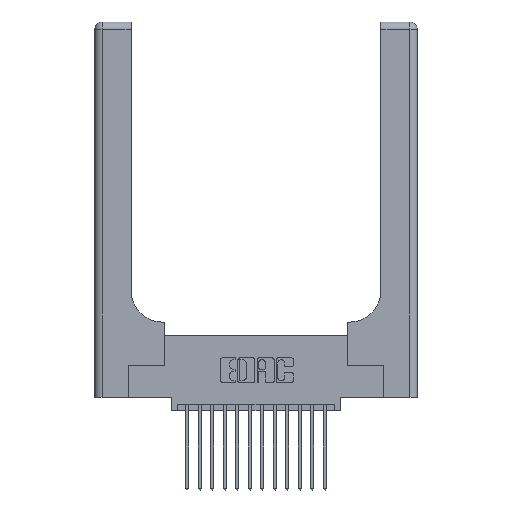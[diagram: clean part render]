
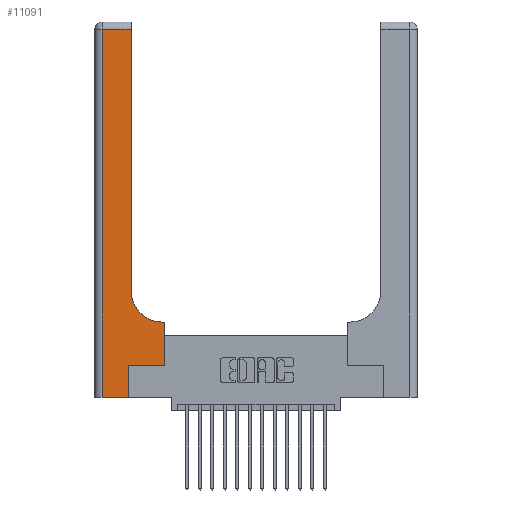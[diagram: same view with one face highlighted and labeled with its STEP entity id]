
A CAD part, top view. The second image highlights one B-rep face of the part: STEP entity #11091.
In plain terms, the highlighted planar face has unit normal (0, 0, 1).
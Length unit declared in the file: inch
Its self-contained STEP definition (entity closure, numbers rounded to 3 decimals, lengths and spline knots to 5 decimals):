
#57 = LINE ( 'NONE', #12612, #15238 ) ;
#309 = LINE ( 'NONE', #1431, #12559 ) ;
#546 = DIRECTION ( 'NONE',  ( -1., 0., 0. ) ) ;
#601 = CARTESIAN_POINT ( 'NONE',  ( 0.06, 0., 0.37 ) ) ;
#1431 = CARTESIAN_POINT ( 'NONE',  ( 0., 0., 0.37 ) ) ;
#1737 = LINE ( 'NONE', #11114, #10131 ) ;
#2006 = VERTEX_POINT ( 'NONE', #17829 ) ;
#2200 = VECTOR ( 'NONE', #17034, 39.37008 ) ;
#2235 = VECTOR ( 'NONE', #14270, 39.37008 ) ;
#2301 = VERTEX_POINT ( 'NONE', #14633 ) ;
#2372 = DIRECTION ( 'NONE',  ( -1., 0., 0. ) ) ;
#2951 = CARTESIAN_POINT ( 'NONE',  ( 0.5415, 0.85, 0.37 ) ) ;
#3018 = VECTOR ( 'NONE', #6677, 39.37008 ) ;
#3206 = ORIENTED_EDGE ( 'NONE', *, *, #6634, .T. ) ;
#3390 = CARTESIAN_POINT ( 'NONE',  ( 0.2915, 3., 0.37 ) ) ;
#3450 = AXIS2_PLACEMENT_3D ( 'NONE', #2951, #13175, #4535 ) ;
#3477 = ORIENTED_EDGE ( 'NONE', *, *, #6862, .T. ) ;
#3519 = LINE ( 'NONE', #5178, #3018 ) ;
#4175 = CARTESIAN_POINT ( 'NONE',  ( 0., 2.94, 0.37 ) ) ;
#4234 = LINE ( 'NONE', #3390, #4718 ) ;
#4363 = EDGE_CURVE ( 'NONE', #2301, #14396, #9798, .T. ) ;
#4377 = AXIS2_PLACEMENT_3D ( 'NONE', #17918, #9528, #546 ) ;
#4535 = DIRECTION ( 'NONE',  ( 1., 0., 0. ) ) ;
#4718 = VECTOR ( 'NONE', #12140, 39.37008 ) ;
#5178 = CARTESIAN_POINT ( 'NONE',  ( 0.269, 0.25, 0.37 ) ) ;
#5514 = LINE ( 'NONE', #12305, #12695 ) ;
#5756 = EDGE_CURVE ( 'NONE', #14396, #9933, #4234, .T. ) ;
#5831 = LINE ( 'NONE', #4175, #2235 ) ;
#6221 = ORIENTED_EDGE ( 'NONE', *, *, #18568, .T. ) ;
#6262 = LINE ( 'NONE', #8596, #2200 ) ;
#6634 = EDGE_CURVE ( 'NONE', #9557, #2301, #57, .T. ) ;
#6677 = DIRECTION ( 'NONE',  ( 1., 0., 0. ) ) ;
#6795 = DIRECTION ( 'NONE',  ( 0., -1., 0. ) ) ;
#6840 = ORIENTED_EDGE ( 'NONE', *, *, #7836, .T. ) ;
#6862 = EDGE_CURVE ( 'NONE', #9350, #18767, #309, .T. ) ;
#7094 = CARTESIAN_POINT ( 'NONE',  ( 0.269, 0., 0.37 ) ) ;
#7340 = EDGE_CURVE ( 'NONE', #9933, #10469, #5831, .T. ) ;
#7836 = EDGE_CURVE ( 'NONE', #10469, #9350, #1737, .T. ) ;
#8004 = CARTESIAN_POINT ( 'NONE',  ( 0.2915, 2.94, 0.37 ) ) ;
#8029 = PLANE ( 'NONE',  #4377 ) ;
#8596 = CARTESIAN_POINT ( 'NONE',  ( 0.5585, 0.25, 0.37 ) ) ;
#9350 = VERTEX_POINT ( 'NONE', #601 ) ;
#9528 = DIRECTION ( 'NONE',  ( 0., 0., -1. ) ) ;
#9545 = VERTEX_POINT ( 'NONE', #10030 ) ;
#9557 = VERTEX_POINT ( 'NONE', #12852 ) ;
#9798 = CIRCLE ( 'NONE', #3450, 0.25 ) ;
#9933 = VERTEX_POINT ( 'NONE', #8004 ) ;
#10030 = CARTESIAN_POINT ( 'NONE',  ( 0.5585, 0.25, 0.37 ) ) ;
#10131 = VECTOR ( 'NONE', #6795, 39.37008 ) ;
#10469 = VERTEX_POINT ( 'NONE', #17763 ) ;
#10500 = ORIENTED_EDGE ( 'NONE', *, *, #4363, .T. ) ;
#11091 = ADVANCED_FACE ( 'NONE', ( #17546 ), #8029, .F. ) ;
#11114 = CARTESIAN_POINT ( 'NONE',  ( 0.06, 3., 0.37 ) ) ;
#11766 = DIRECTION ( 'NONE',  ( 1., 0., 0. ) ) ;
#12140 = DIRECTION ( 'NONE',  ( 0., 1., 0. ) ) ;
#12305 = CARTESIAN_POINT ( 'NONE',  ( 0.269, 0., 0.37 ) ) ;
#12357 = EDGE_LOOP ( 'NONE', ( #15411, #16146, #6840, #3477, #6221, #12609, #15898, #3206, #10500 ) ) ;
#12559 = VECTOR ( 'NONE', #11766, 39.37008 ) ;
#12609 = ORIENTED_EDGE ( 'NONE', *, *, #13800, .T. ) ;
#12612 = CARTESIAN_POINT ( 'NONE',  ( 0.2915, 0.6, 0.37 ) ) ;
#12695 = VECTOR ( 'NONE', #13743, 39.37008 ) ;
#12852 = CARTESIAN_POINT ( 'NONE',  ( 0.5585, 0.6, 0.37 ) ) ;
#13175 = DIRECTION ( 'NONE',  ( 0., 0., -1. ) ) ;
#13743 = DIRECTION ( 'NONE',  ( 0., 1., 0. ) ) ;
#13800 = EDGE_CURVE ( 'NONE', #2006, #9545, #3519, .T. ) ;
#14270 = DIRECTION ( 'NONE',  ( -1., 0., 0. ) ) ;
#14396 = VERTEX_POINT ( 'NONE', #17704 ) ;
#14633 = CARTESIAN_POINT ( 'NONE',  ( 0.5415, 0.6, 0.37 ) ) ;
#15238 = VECTOR ( 'NONE', #2372, 39.37008 ) ;
#15411 = ORIENTED_EDGE ( 'NONE', *, *, #5756, .T. ) ;
#15898 = ORIENTED_EDGE ( 'NONE', *, *, #17388, .T. ) ;
#16146 = ORIENTED_EDGE ( 'NONE', *, *, #7340, .T. ) ;
#17034 = DIRECTION ( 'NONE',  ( 0., 1., 0. ) ) ;
#17388 = EDGE_CURVE ( 'NONE', #9545, #9557, #6262, .T. ) ;
#17546 = FACE_OUTER_BOUND ( 'NONE', #12357, .T. ) ;
#17704 = CARTESIAN_POINT ( 'NONE',  ( 0.2915, 0.85, 0.37 ) ) ;
#17763 = CARTESIAN_POINT ( 'NONE',  ( 0.06, 2.94, 0.37 ) ) ;
#17829 = CARTESIAN_POINT ( 'NONE',  ( 0.269, 0.25, 0.37 ) ) ;
#17918 = CARTESIAN_POINT ( 'NONE',  ( 0., 3., 0.37 ) ) ;
#18568 = EDGE_CURVE ( 'NONE', #18767, #2006, #5514, .T. ) ;
#18767 = VERTEX_POINT ( 'NONE', #7094 ) ;
